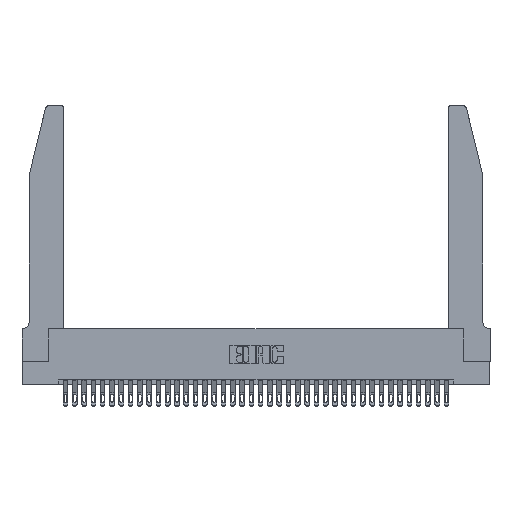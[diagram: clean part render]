
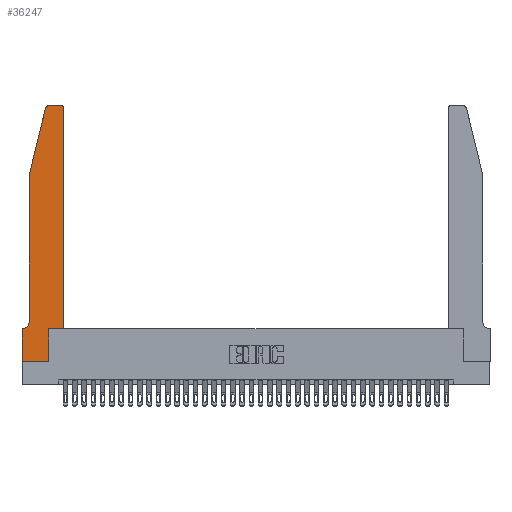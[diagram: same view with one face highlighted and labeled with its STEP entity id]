
A CAD part, top view. The second image highlights one B-rep face of the part: STEP entity #36247.
In plain terms, the highlighted planar face has unit normal (0, 0, 1).
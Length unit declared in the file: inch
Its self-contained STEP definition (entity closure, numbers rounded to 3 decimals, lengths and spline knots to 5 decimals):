
#275 = CARTESIAN_POINT ( 'NONE',  ( 0.4505, 0.35, 0.37 ) ) ;
#1549 = CARTESIAN_POINT ( 'NONE',  ( 0.0755, 0.35, 0.37 ) ) ;
#2449 = EDGE_CURVE ( 'NONE', #16322, #8318, #5247, .T. ) ;
#2640 = CARTESIAN_POINT ( 'NONE',  ( 0.0055, 0.35, 0.37 ) ) ;
#2678 = LINE ( 'NONE', #7627, #25309 ) ;
#3055 = AXIS2_PLACEMENT_3D ( 'NONE', #31576, #14138, #34490 ) ;
#3173 = LINE ( 'NONE', #275, #24869 ) ;
#3297 = CIRCLE ( 'NONE', #14445, 0.03 ) ;
#3488 = VERTEX_POINT ( 'NONE', #11762 ) ;
#4432 = CARTESIAN_POINT ( 'NONE',  ( 0.4505, 2.72, 0.37 ) ) ;
#4733 = EDGE_CURVE ( 'NONE', #15413, #17207, #16729, .T. ) ;
#4978 = ORIENTED_EDGE ( 'NONE', *, *, #8582, .T. ) ;
#5247 = LINE ( 'NONE', #24754, #27797 ) ;
#5767 = CARTESIAN_POINT ( 'NONE',  ( 0.0755, 2., 0.37 ) ) ;
#6057 = EDGE_CURVE ( 'NONE', #8318, #9896, #9683, .T. ) ;
#6156 = VERTEX_POINT ( 'NONE', #30879 ) ;
#6346 = ORIENTED_EDGE ( 'NONE', *, *, #7167, .T. ) ;
#6586 = CARTESIAN_POINT ( 'NONE',  ( 0., 0.35, 0.37 ) ) ;
#7037 = DIRECTION ( 'NONE',  ( 0., 0., 1. ) ) ;
#7167 = EDGE_CURVE ( 'NONE', #8540, #23092, #3173, .T. ) ;
#7203 = EDGE_CURVE ( 'NONE', #3488, #8540, #17161, .T. ) ;
#7234 = CARTESIAN_POINT ( 'NONE',  ( 0.2865, 0.35, 0.37 ) ) ;
#7297 = ORIENTED_EDGE ( 'NONE', *, *, #7376, .T. ) ;
#7376 = EDGE_CURVE ( 'NONE', #17207, #38008, #2678, .T. ) ;
#7470 = FACE_OUTER_BOUND ( 'NONE', #20499, .T. ) ;
#7627 = CARTESIAN_POINT ( 'NONE',  ( 0., 0., 0.37 ) ) ;
#8318 = VERTEX_POINT ( 'NONE', #26811 ) ;
#8347 = CARTESIAN_POINT ( 'NONE',  ( 0.4205, 2.72, 0.37 ) ) ;
#8540 = VERTEX_POINT ( 'NONE', #13125 ) ;
#8582 = EDGE_CURVE ( 'NONE', #25769, #6156, #12908, .T. ) ;
#8965 = CARTESIAN_POINT ( 'NONE',  ( 0., 0., 0.37 ) ) ;
#9356 = CARTESIAN_POINT ( 'NONE',  ( 0.4505, 0.35, 0.37 ) ) ;
#9683 = CIRCLE ( 'NONE', #23599, 0.03 ) ;
#9896 = VERTEX_POINT ( 'NONE', #36561 ) ;
#10120 = DIRECTION ( 'NONE',  ( 0., 1., 0. ) ) ;
#10127 = EDGE_CURVE ( 'NONE', #6156, #17166, #26938, .T. ) ;
#10340 = LINE ( 'NONE', #5767, #32703 ) ;
#11071 = VECTOR ( 'NONE', #10120, 39.37008 ) ;
#11347 = DIRECTION ( 'NONE',  ( 1., 0., 0. ) ) ;
#11632 = EDGE_CURVE ( 'NONE', #9896, #25769, #10340, .T. ) ;
#11762 = CARTESIAN_POINT ( 'NONE',  ( 0.2865, 0.35, 0.37 ) ) ;
#11978 = VECTOR ( 'NONE', #25194, 39.37008 ) ;
#12411 = ORIENTED_EDGE ( 'NONE', *, *, #11632, .T. ) ;
#12908 = LINE ( 'NONE', #27115, #17984 ) ;
#13125 = CARTESIAN_POINT ( 'NONE',  ( 0.4505, 0.35, 0.37 ) ) ;
#13810 = LINE ( 'NONE', #1549, #11978 ) ;
#13959 = VECTOR ( 'NONE', #17215, 39.37008 ) ;
#14105 = ORIENTED_EDGE ( 'NONE', *, *, #6057, .T. ) ;
#14138 = DIRECTION ( 'NONE',  ( 0., 0., 1. ) ) ;
#14397 = DIRECTION ( 'NONE',  ( 0., 0., -1. ) ) ;
#14445 = AXIS2_PLACEMENT_3D ( 'NONE', #8347, #28810, #11347 ) ;
#15111 = ORIENTED_EDGE ( 'NONE', *, *, #4733, .T. ) ;
#15413 = VERTEX_POINT ( 'NONE', #6586 ) ;
#15930 = ORIENTED_EDGE ( 'NONE', *, *, #2449, .T. ) ;
#16235 = VECTOR ( 'NONE', #24074, 39.37008 ) ;
#16322 = VERTEX_POINT ( 'NONE', #28211 ) ;
#16335 = CARTESIAN_POINT ( 'NONE',  ( 0.2865, 0., 0.37 ) ) ;
#16729 = LINE ( 'NONE', #34608, #13959 ) ;
#17161 = LINE ( 'NONE', #9356, #16235 ) ;
#17166 = VERTEX_POINT ( 'NONE', #2640 ) ;
#17207 = VERTEX_POINT ( 'NONE', #8965 ) ;
#17215 = DIRECTION ( 'NONE',  ( 0., -1., 0. ) ) ;
#17724 = DIRECTION ( 'NONE',  ( -0.239, -0.971, 0. ) ) ;
#17984 = VECTOR ( 'NONE', #30039, 39.37008 ) ;
#19811 = LINE ( 'NONE', #7234, #11071 ) ;
#19899 = PLANE ( 'NONE',  #3055 ) ;
#20046 = EDGE_CURVE ( 'NONE', #23092, #16322, #3297, .T. ) ;
#20499 = EDGE_LOOP ( 'NONE', ( #15930, #14105, #12411, #4978, #29078, #22689, #15111, #7297, #28781, #25912, #6346, #26312 ) ) ;
#22689 = ORIENTED_EDGE ( 'NONE', *, *, #23115, .T. ) ;
#23092 = VERTEX_POINT ( 'NONE', #4432 ) ;
#23115 = EDGE_CURVE ( 'NONE', #17166, #15413, #13810, .T. ) ;
#23599 = AXIS2_PLACEMENT_3D ( 'NONE', #24653, #7037, #27571 ) ;
#23952 = DIRECTION ( 'NONE',  ( 0., 1., 0. ) ) ;
#24074 = DIRECTION ( 'NONE',  ( 1., 0., 0. ) ) ;
#24644 = CARTESIAN_POINT ( 'NONE',  ( 0.0755, 2., 0.37 ) ) ;
#24653 = CARTESIAN_POINT ( 'NONE',  ( 0.284, 2.72, 0.37 ) ) ;
#24754 = CARTESIAN_POINT ( 'NONE',  ( 0.2605, 2.75, 0.37 ) ) ;
#24869 = VECTOR ( 'NONE', #23952, 39.37008 ) ;
#25194 = DIRECTION ( 'NONE',  ( -1., 0., 0. ) ) ;
#25309 = VECTOR ( 'NONE', #28122, 39.37008 ) ;
#25769 = VERTEX_POINT ( 'NONE', #24644 ) ;
#25912 = ORIENTED_EDGE ( 'NONE', *, *, #7203, .T. ) ;
#26312 = ORIENTED_EDGE ( 'NONE', *, *, #20046, .T. ) ;
#26811 = CARTESIAN_POINT ( 'NONE',  ( 0.284, 2.75, 0.37 ) ) ;
#26938 = CIRCLE ( 'NONE', #35131, 0.07 ) ;
#27115 = CARTESIAN_POINT ( 'NONE',  ( 0.0755, 2., 0.37 ) ) ;
#27571 = DIRECTION ( 'NONE',  ( 1., 0., 0. ) ) ;
#27682 = DIRECTION ( 'NONE',  ( -1., 0., 0. ) ) ;
#27797 = VECTOR ( 'NONE', #27682, 39.37008 ) ;
#28122 = DIRECTION ( 'NONE',  ( 1., 0., 0. ) ) ;
#28211 = CARTESIAN_POINT ( 'NONE',  ( 0.4205, 2.75, 0.37 ) ) ;
#28781 = ORIENTED_EDGE ( 'NONE', *, *, #37959, .T. ) ;
#28810 = DIRECTION ( 'NONE',  ( 0., 0., 1. ) ) ;
#29078 = ORIENTED_EDGE ( 'NONE', *, *, #10127, .T. ) ;
#30039 = DIRECTION ( 'NONE',  ( 0., -1., 0. ) ) ;
#30879 = CARTESIAN_POINT ( 'NONE',  ( 0.0755, 0.42, 0.37 ) ) ;
#31576 = CARTESIAN_POINT ( 'NONE',  ( 0., 0.35, 0.37 ) ) ;
#31837 = CARTESIAN_POINT ( 'NONE',  ( 0.0055, 0.42, 0.37 ) ) ;
#32703 = VECTOR ( 'NONE', #17724, 39.37008 ) ;
#34490 = DIRECTION ( 'NONE',  ( 1., 0., 0. ) ) ;
#34608 = CARTESIAN_POINT ( 'NONE',  ( 0., 0., 0.37 ) ) ;
#34762 = DIRECTION ( 'NONE',  ( -1., 0., 0. ) ) ;
#35131 = AXIS2_PLACEMENT_3D ( 'NONE', #31837, #14397, #34762 ) ;
#36247 = ADVANCED_FACE ( 'NONE', ( #7470 ), #19899, .T. ) ;
#36561 = CARTESIAN_POINT ( 'NONE',  ( 0.25487, 2.72718, 0.37 ) ) ;
#37959 = EDGE_CURVE ( 'NONE', #38008, #3488, #19811, .T. ) ;
#38008 = VERTEX_POINT ( 'NONE', #16335 ) ;
